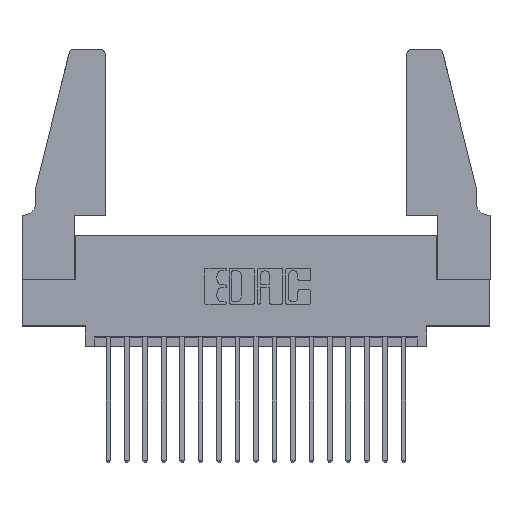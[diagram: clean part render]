
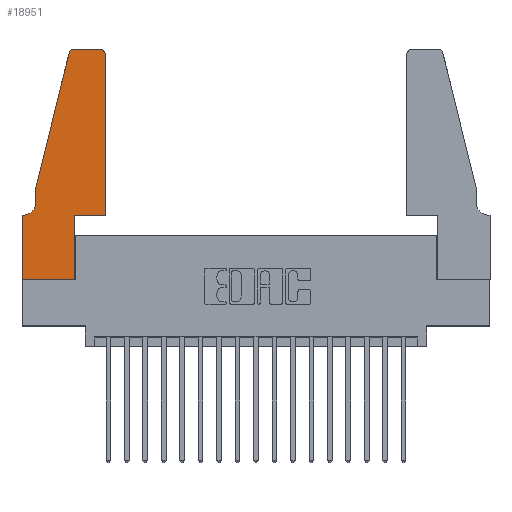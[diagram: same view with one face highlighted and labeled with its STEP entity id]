
A CAD part, top view. The second image highlights one B-rep face of the part: STEP entity #18951.
In plain terms, the highlighted planar face has unit normal (0, 0, 1).
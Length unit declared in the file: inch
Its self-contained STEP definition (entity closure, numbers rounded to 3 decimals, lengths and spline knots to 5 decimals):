
#421 = LINE ( 'NONE', #4216, #11841 ) ;
#451 = CARTESIAN_POINT ( 'NONE',  ( 0.4505, 1.22, 0.37 ) ) ;
#494 = EDGE_CURVE ( 'NONE', #12743, #501, #421, .T. ) ;
#501 = VERTEX_POINT ( 'NONE', #8570 ) ;
#741 = ORIENTED_EDGE ( 'NONE', *, *, #5077, .T. ) ;
#1185 = EDGE_CURVE ( 'NONE', #16065, #1958, #5699, .T. ) ;
#1263 = CARTESIAN_POINT ( 'NONE',  ( 0.0055, 0.35, 0.37 ) ) ;
#1579 = ORIENTED_EDGE ( 'NONE', *, *, #12882, .T. ) ;
#1850 = LINE ( 'NONE', #2668, #14034 ) ;
#1882 = VECTOR ( 'NONE', #16827, 39.37008 ) ;
#1884 = DIRECTION ( 'NONE',  ( 1., 0., 0. ) ) ;
#1958 = VERTEX_POINT ( 'NONE', #451 ) ;
#2307 = DIRECTION ( 'NONE',  ( -1., 0., 0. ) ) ;
#2668 = CARTESIAN_POINT ( 'NONE',  ( 0.0755, 0.5, 0.37 ) ) ;
#2676 = ORIENTED_EDGE ( 'NONE', *, *, #9370, .T. ) ;
#2792 = FACE_OUTER_BOUND ( 'NONE', #17326, .T. ) ;
#2898 = VERTEX_POINT ( 'NONE', #13386 ) ;
#3020 = VERTEX_POINT ( 'NONE', #1263 ) ;
#3214 = VERTEX_POINT ( 'NONE', #14880 ) ;
#3377 = AXIS2_PLACEMENT_3D ( 'NONE', #7642, #17667, #9098 ) ;
#3435 = ORIENTED_EDGE ( 'NONE', *, *, #5362, .T. ) ;
#3645 = LINE ( 'NONE', #10164, #11442 ) ;
#3856 = CIRCLE ( 'NONE', #14430, 0.03 ) ;
#4216 = CARTESIAN_POINT ( 'NONE',  ( 0.0755, 0.5, 0.37 ) ) ;
#4334 = VERTEX_POINT ( 'NONE', #18700 ) ;
#4916 = DIRECTION ( 'NONE',  ( 1., 0., 0. ) ) ;
#5077 = EDGE_CURVE ( 'NONE', #12821, #10236, #3645, .T. ) ;
#5362 = EDGE_CURVE ( 'NONE', #16331, #16065, #17939, .T. ) ;
#5485 = AXIS2_PLACEMENT_3D ( 'NONE', #12127, #10760, #1884 ) ;
#5548 = CARTESIAN_POINT ( 'NONE',  ( 0., 0., 0.37 ) ) ;
#5657 = CIRCLE ( 'NONE', #11349, 0.03 ) ;
#5699 = LINE ( 'NONE', #10073, #12941 ) ;
#5717 = VECTOR ( 'NONE', #16653, 39.37008 ) ;
#5755 = DIRECTION ( 'NONE',  ( 0., 1., 0. ) ) ;
#6220 = DIRECTION ( 'NONE',  ( 0., 0., 1. ) ) ;
#6415 = CARTESIAN_POINT ( 'NONE',  ( 0.4505, 0.35, 0.37 ) ) ;
#6456 = VECTOR ( 'NONE', #4916, 39.37008 ) ;
#6665 = CARTESIAN_POINT ( 'NONE',  ( 0.2865, 0.35, 0.37 ) ) ;
#6767 = CARTESIAN_POINT ( 'NONE',  ( 0., 0., 0.37 ) ) ;
#6835 = ORIENTED_EDGE ( 'NONE', *, *, #10398, .T. ) ;
#7028 = CARTESIAN_POINT ( 'NONE',  ( 0.4205, 1.22, 0.37 ) ) ;
#7164 = ORIENTED_EDGE ( 'NONE', *, *, #17131, .T. ) ;
#7402 = CARTESIAN_POINT ( 'NONE',  ( 0.284, 1.25, 0.37 ) ) ;
#7642 = CARTESIAN_POINT ( 'NONE',  ( 0.0055, 0.42, 0.37 ) ) ;
#7993 = EDGE_CURVE ( 'NONE', #4334, #15016, #13862, .T. ) ;
#8064 = CARTESIAN_POINT ( 'NONE',  ( 0.2605, 1.25, 0.37 ) ) ;
#8358 = VECTOR ( 'NONE', #18562, 39.37008 ) ;
#8498 = DIRECTION ( 'NONE',  ( 1., 0., 0. ) ) ;
#8570 = CARTESIAN_POINT ( 'NONE',  ( 0.0755, 0.42, 0.37 ) ) ;
#8822 = LINE ( 'NONE', #9989, #8358 ) ;
#9098 = DIRECTION ( 'NONE',  ( -1., 0., 0. ) ) ;
#9370 = EDGE_CURVE ( 'NONE', #2898, #12821, #12719, .T. ) ;
#9754 = CARTESIAN_POINT ( 'NONE',  ( 0.0755, 0.5, 0.37 ) ) ;
#9989 = CARTESIAN_POINT ( 'NONE',  ( 0.2865, 0.35, 0.37 ) ) ;
#10073 = CARTESIAN_POINT ( 'NONE',  ( 0.4505, 0.35, 0.37 ) ) ;
#10164 = CARTESIAN_POINT ( 'NONE',  ( 0., 0., 0.37 ) ) ;
#10236 = VERTEX_POINT ( 'NONE', #17359 ) ;
#10398 = EDGE_CURVE ( 'NONE', #15016, #3214, #5657, .T. ) ;
#10760 = DIRECTION ( 'NONE',  ( 0., 0., 1. ) ) ;
#11220 = ORIENTED_EDGE ( 'NONE', *, *, #15318, .T. ) ;
#11349 = AXIS2_PLACEMENT_3D ( 'NONE', #14862, #6220, #16287 ) ;
#11381 = ORIENTED_EDGE ( 'NONE', *, *, #494, .T. ) ;
#11442 = VECTOR ( 'NONE', #11539, 39.37008 ) ;
#11492 = DIRECTION ( 'NONE',  ( -0.239, -0.971, 0. ) ) ;
#11539 = DIRECTION ( 'NONE',  ( 1., 0., 0. ) ) ;
#11593 = CARTESIAN_POINT ( 'NONE',  ( 0.4505, 0.35, 0.37 ) ) ;
#11841 = VECTOR ( 'NONE', #14476, 39.37008 ) ;
#12127 = CARTESIAN_POINT ( 'NONE',  ( 0., 0.35, 0.37 ) ) ;
#12609 = CARTESIAN_POINT ( 'NONE',  ( 0.0755, 0.35, 0.37 ) ) ;
#12719 = LINE ( 'NONE', #6767, #1882 ) ;
#12743 = VERTEX_POINT ( 'NONE', #9754 ) ;
#12821 = VERTEX_POINT ( 'NONE', #5548 ) ;
#12882 = EDGE_CURVE ( 'NONE', #3214, #12743, #1850, .T. ) ;
#12908 = CIRCLE ( 'NONE', #3377, 0.07 ) ;
#12941 = VECTOR ( 'NONE', #5755, 39.37008 ) ;
#13110 = ORIENTED_EDGE ( 'NONE', *, *, #7993, .T. ) ;
#13386 = CARTESIAN_POINT ( 'NONE',  ( 0., 0.35, 0.37 ) ) ;
#13713 = VECTOR ( 'NONE', #2307, 39.37008 ) ;
#13767 = EDGE_CURVE ( 'NONE', #501, #3020, #12908, .T. ) ;
#13862 = LINE ( 'NONE', #8064, #5717 ) ;
#14034 = VECTOR ( 'NONE', #11492, 39.37008 ) ;
#14171 = LINE ( 'NONE', #12609, #13713 ) ;
#14430 = AXIS2_PLACEMENT_3D ( 'NONE', #7028, #17068, #8498 ) ;
#14476 = DIRECTION ( 'NONE',  ( 0., -1., 0. ) ) ;
#14862 = CARTESIAN_POINT ( 'NONE',  ( 0.284, 1.22, 0.37 ) ) ;
#14880 = CARTESIAN_POINT ( 'NONE',  ( 0.25487, 1.22718, 0.37 ) ) ;
#15016 = VERTEX_POINT ( 'NONE', #7402 ) ;
#15318 = EDGE_CURVE ( 'NONE', #10236, #16331, #8822, .T. ) ;
#15875 = EDGE_CURVE ( 'NONE', #3020, #2898, #14171, .T. ) ;
#16065 = VERTEX_POINT ( 'NONE', #11593 ) ;
#16189 = ORIENTED_EDGE ( 'NONE', *, *, #1185, .T. ) ;
#16287 = DIRECTION ( 'NONE',  ( 1., 0., 0. ) ) ;
#16331 = VERTEX_POINT ( 'NONE', #6665 ) ;
#16653 = DIRECTION ( 'NONE',  ( -1., 0., 0. ) ) ;
#16827 = DIRECTION ( 'NONE',  ( 0., -1., 0. ) ) ;
#16963 = ORIENTED_EDGE ( 'NONE', *, *, #15875, .T. ) ;
#16996 = ORIENTED_EDGE ( 'NONE', *, *, #13767, .T. ) ;
#17068 = DIRECTION ( 'NONE',  ( 0., 0., 1. ) ) ;
#17131 = EDGE_CURVE ( 'NONE', #1958, #4334, #3856, .T. ) ;
#17326 = EDGE_LOOP ( 'NONE', ( #13110, #6835, #1579, #11381, #16996, #16963, #2676, #741, #11220, #3435, #16189, #7164 ) ) ;
#17359 = CARTESIAN_POINT ( 'NONE',  ( 0.2865, 0., 0.37 ) ) ;
#17667 = DIRECTION ( 'NONE',  ( 0., 0., -1. ) ) ;
#17898 = PLANE ( 'NONE',  #5485 ) ;
#17939 = LINE ( 'NONE', #6415, #6456 ) ;
#18562 = DIRECTION ( 'NONE',  ( 0., 1., 0. ) ) ;
#18700 = CARTESIAN_POINT ( 'NONE',  ( 0.4205, 1.25, 0.37 ) ) ;
#18951 = ADVANCED_FACE ( 'NONE', ( #2792 ), #17898, .T. ) ;
